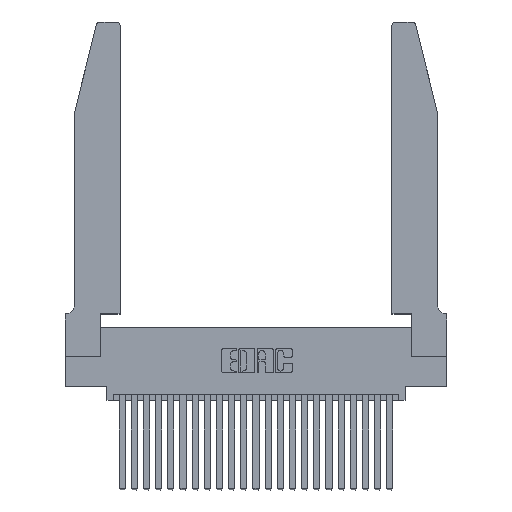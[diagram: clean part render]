
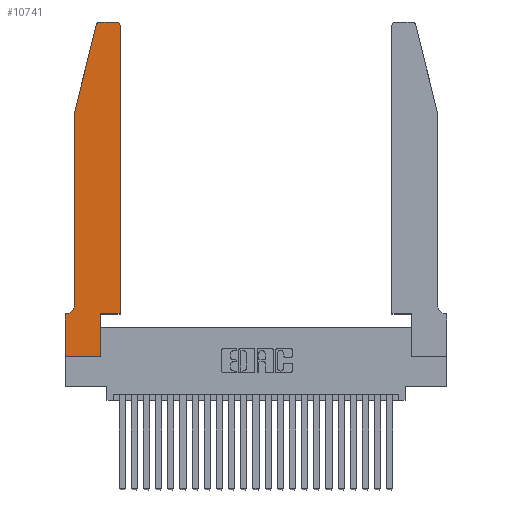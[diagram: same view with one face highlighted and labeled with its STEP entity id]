
A CAD part, top view. The second image highlights one B-rep face of the part: STEP entity #10741.
In plain terms, the highlighted planar face has unit normal (0, 0, 1).
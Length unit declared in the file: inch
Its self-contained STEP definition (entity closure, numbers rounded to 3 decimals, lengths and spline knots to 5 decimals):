
#339 = PLANE ( 'NONE',  #15857 ) ;
#395 = CARTESIAN_POINT ( 'NONE',  ( 0.2865, 0.35, 0.37 ) ) ;
#405 = LINE ( 'NONE', #18853, #5812 ) ;
#663 = VERTEX_POINT ( 'NONE', #3081 ) ;
#785 = LINE ( 'NONE', #16597, #5539 ) ;
#1483 = CARTESIAN_POINT ( 'NONE',  ( 0.2865, 0., 0.37 ) ) ;
#2158 = CARTESIAN_POINT ( 'NONE',  ( 0.0755, 0.35, 0.37 ) ) ;
#2374 = CIRCLE ( 'NONE', #16867, 0.03 ) ;
#2404 = DIRECTION ( 'NONE',  ( 1., 0., 0. ) ) ;
#2600 = LINE ( 'NONE', #21835, #12688 ) ;
#2668 = LINE ( 'NONE', #22787, #12755 ) ;
#2792 = DIRECTION ( 'NONE',  ( -1., 0., 0. ) ) ;
#2916 = EDGE_CURVE ( 'NONE', #11554, #663, #7277, .T. ) ;
#3081 = CARTESIAN_POINT ( 'NONE',  ( 0.0055, 0.35, 0.37 ) ) ;
#3089 = LINE ( 'NONE', #10215, #13768 ) ;
#3132 = VERTEX_POINT ( 'NONE', #395 ) ;
#3164 = VERTEX_POINT ( 'NONE', #12158 ) ;
#3284 = CARTESIAN_POINT ( 'NONE',  ( 0.284, 2.75, 0.37 ) ) ;
#3497 = CARTESIAN_POINT ( 'NONE',  ( 0.4205, 2.72, 0.37 ) ) ;
#3881 = EDGE_CURVE ( 'NONE', #10102, #24000, #16688, .T. ) ;
#4022 = DIRECTION ( 'NONE',  ( 0., 1., 0. ) ) ;
#4084 = EDGE_CURVE ( 'NONE', #16667, #20565, #2374, .T. ) ;
#4979 = VERTEX_POINT ( 'NONE', #1483 ) ;
#5282 = DIRECTION ( 'NONE',  ( 1., 0., 0. ) ) ;
#5395 = AXIS2_PLACEMENT_3D ( 'NONE', #3497, #17349, #5518 ) ;
#5518 = DIRECTION ( 'NONE',  ( 1., 0., 0. ) ) ;
#5539 = VECTOR ( 'NONE', #2792, 39.37008 ) ;
#5672 = CARTESIAN_POINT ( 'NONE',  ( 0.4505, 2.72, 0.37 ) ) ;
#5742 = EDGE_CURVE ( 'NONE', #663, #3164, #8638, .T. ) ;
#5786 = EDGE_CURVE ( 'NONE', #4979, #3132, #2600, .T. ) ;
#5812 = VECTOR ( 'NONE', #7179, 39.37008 ) ;
#5831 = CARTESIAN_POINT ( 'NONE',  ( 0.0055, 0.42, 0.37 ) ) ;
#5846 = CIRCLE ( 'NONE', #5395, 0.03 ) ;
#5925 = ORIENTED_EDGE ( 'NONE', *, *, #23328, .T. ) ;
#6321 = DIRECTION ( 'NONE',  ( 0., 1., 0. ) ) ;
#6552 = DIRECTION ( 'NONE',  ( -1., 0., 0. ) ) ;
#6669 = ORIENTED_EDGE ( 'NONE', *, *, #24750, .T. ) ;
#6944 = DIRECTION ( 'NONE',  ( 0., 0., -1. ) ) ;
#7179 = DIRECTION ( 'NONE',  ( 0., -1., 0. ) ) ;
#7266 = EDGE_LOOP ( 'NONE', ( #10702, #8022, #6669, #8724, #16457, #17400, #5925, #21755, #13019, #21633, #8965, #22259 ) ) ;
#7277 = CIRCLE ( 'NONE', #25054, 0.07 ) ;
#7396 = CARTESIAN_POINT ( 'NONE',  ( 0., 0., 0.37 ) ) ;
#8022 = ORIENTED_EDGE ( 'NONE', *, *, #4084, .T. ) ;
#8423 = CARTESIAN_POINT ( 'NONE',  ( 0.4205, 2.75, 0.37 ) ) ;
#8638 = LINE ( 'NONE', #2158, #13910 ) ;
#8724 = ORIENTED_EDGE ( 'NONE', *, *, #24381, .T. ) ;
#8803 = DIRECTION ( 'NONE',  ( 0., 0., 1. ) ) ;
#8965 = ORIENTED_EDGE ( 'NONE', *, *, #3881, .T. ) ;
#9607 = LINE ( 'NONE', #12937, #19275 ) ;
#10035 = CARTESIAN_POINT ( 'NONE',  ( 0.4505, 0.35, 0.37 ) ) ;
#10102 = VERTEX_POINT ( 'NONE', #18173 ) ;
#10215 = CARTESIAN_POINT ( 'NONE',  ( 0., 0., 0.37 ) ) ;
#10454 = CARTESIAN_POINT ( 'NONE',  ( 0., 0.35, 0.37 ) ) ;
#10702 = ORIENTED_EDGE ( 'NONE', *, *, #12020, .T. ) ;
#10741 = ADVANCED_FACE ( 'NONE', ( #13155 ), #339, .T. ) ;
#11546 = VECTOR ( 'NONE', #4022, 39.37008 ) ;
#11554 = VERTEX_POINT ( 'NONE', #15208 ) ;
#12020 = EDGE_CURVE ( 'NONE', #19987, #16667, #785, .T. ) ;
#12158 = CARTESIAN_POINT ( 'NONE',  ( 0., 0.35, 0.37 ) ) ;
#12266 = EDGE_CURVE ( 'NONE', #24000, #19987, #5846, .T. ) ;
#12688 = VECTOR ( 'NONE', #6321, 39.37008 ) ;
#12755 = VECTOR ( 'NONE', #5282, 39.37008 ) ;
#12937 = CARTESIAN_POINT ( 'NONE',  ( 0.0755, 2., 0.37 ) ) ;
#13019 = ORIENTED_EDGE ( 'NONE', *, *, #5786, .T. ) ;
#13155 = FACE_OUTER_BOUND ( 'NONE', #7266, .T. ) ;
#13768 = VECTOR ( 'NONE', #23568, 39.37008 ) ;
#13910 = VECTOR ( 'NONE', #16094, 39.37008 ) ;
#14399 = DIRECTION ( 'NONE',  ( 0., 0., 1. ) ) ;
#14882 = DIRECTION ( 'NONE',  ( 0., -1., 0. ) ) ;
#15208 = CARTESIAN_POINT ( 'NONE',  ( 0.0755, 0.42, 0.37 ) ) ;
#15857 = AXIS2_PLACEMENT_3D ( 'NONE', #10454, #14399, #2404 ) ;
#16000 = VECTOR ( 'NONE', #17859, 39.37008 ) ;
#16019 = VERTEX_POINT ( 'NONE', #7396 ) ;
#16094 = DIRECTION ( 'NONE',  ( -1., 0., 0. ) ) ;
#16457 = ORIENTED_EDGE ( 'NONE', *, *, #2916, .T. ) ;
#16597 = CARTESIAN_POINT ( 'NONE',  ( 0.2605, 2.75, 0.37 ) ) ;
#16667 = VERTEX_POINT ( 'NONE', #3284 ) ;
#16688 = LINE ( 'NONE', #10035, #11546 ) ;
#16867 = AXIS2_PLACEMENT_3D ( 'NONE', #20360, #8803, #22236 ) ;
#17349 = DIRECTION ( 'NONE',  ( 0., 0., 1. ) ) ;
#17400 = ORIENTED_EDGE ( 'NONE', *, *, #5742, .T. ) ;
#17530 = EDGE_CURVE ( 'NONE', #16019, #4979, #3089, .T. ) ;
#17859 = DIRECTION ( 'NONE',  ( -0.239, -0.971, 0. ) ) ;
#18173 = CARTESIAN_POINT ( 'NONE',  ( 0.4505, 0.35, 0.37 ) ) ;
#18853 = CARTESIAN_POINT ( 'NONE',  ( 0., 0., 0.37 ) ) ;
#19275 = VECTOR ( 'NONE', #14882, 39.37008 ) ;
#19651 = CARTESIAN_POINT ( 'NONE',  ( 0.0755, 2., 0.37 ) ) ;
#19662 = CARTESIAN_POINT ( 'NONE',  ( 0.25487, 2.72718, 0.37 ) ) ;
#19987 = VERTEX_POINT ( 'NONE', #8423 ) ;
#20335 = EDGE_CURVE ( 'NONE', #3132, #10102, #2668, .T. ) ;
#20360 = CARTESIAN_POINT ( 'NONE',  ( 0.284, 2.72, 0.37 ) ) ;
#20565 = VERTEX_POINT ( 'NONE', #19662 ) ;
#21011 = LINE ( 'NONE', #19651, #16000 ) ;
#21633 = ORIENTED_EDGE ( 'NONE', *, *, #20335, .T. ) ;
#21755 = ORIENTED_EDGE ( 'NONE', *, *, #17530, .T. ) ;
#21835 = CARTESIAN_POINT ( 'NONE',  ( 0.2865, 0.35, 0.37 ) ) ;
#22236 = DIRECTION ( 'NONE',  ( 1., 0., 0. ) ) ;
#22259 = ORIENTED_EDGE ( 'NONE', *, *, #12266, .T. ) ;
#22747 = CARTESIAN_POINT ( 'NONE',  ( 0.0755, 2., 0.37 ) ) ;
#22787 = CARTESIAN_POINT ( 'NONE',  ( 0.4505, 0.35, 0.37 ) ) ;
#23328 = EDGE_CURVE ( 'NONE', #3164, #16019, #405, .T. ) ;
#23568 = DIRECTION ( 'NONE',  ( 1., 0., 0. ) ) ;
#24000 = VERTEX_POINT ( 'NONE', #5672 ) ;
#24381 = EDGE_CURVE ( 'NONE', #25167, #11554, #9607, .T. ) ;
#24750 = EDGE_CURVE ( 'NONE', #20565, #25167, #21011, .T. ) ;
#25054 = AXIS2_PLACEMENT_3D ( 'NONE', #5831, #6944, #6552 ) ;
#25167 = VERTEX_POINT ( 'NONE', #22747 ) ;
